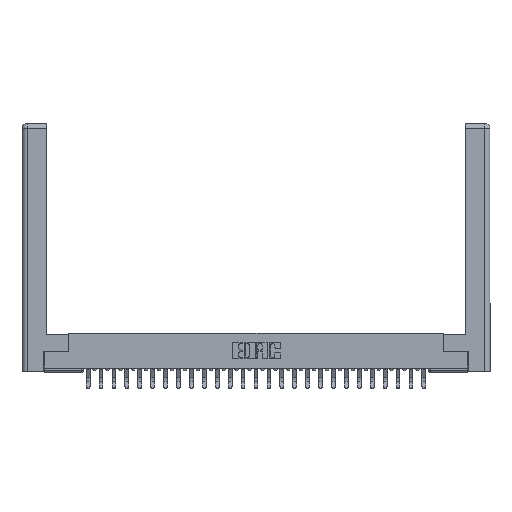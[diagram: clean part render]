
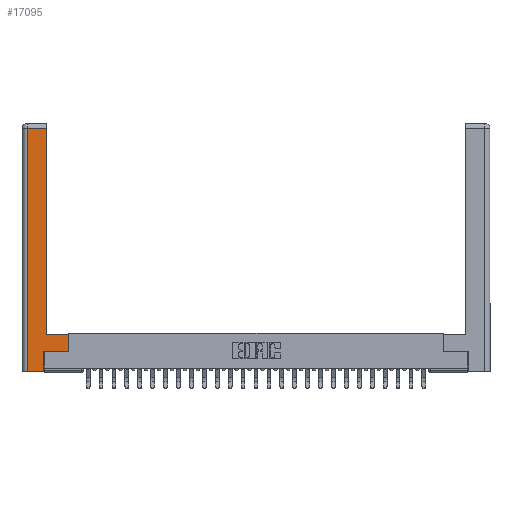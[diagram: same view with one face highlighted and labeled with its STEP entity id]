
A CAD part, top view. The second image highlights one B-rep face of the part: STEP entity #17095.
In plain terms, the highlighted planar face has unit normal (0, 0, 1).
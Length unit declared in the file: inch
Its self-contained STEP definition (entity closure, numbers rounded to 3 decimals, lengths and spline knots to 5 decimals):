
#270 = VECTOR ( 'NONE', #26893, 39.37008 ) ;
#535 = LINE ( 'NONE', #22062, #9933 ) ;
#994 = EDGE_CURVE ( 'NONE', #13343, #8390, #21344, .T. ) ;
#1334 = LINE ( 'NONE', #6790, #270 ) ;
#2785 = CARTESIAN_POINT ( 'NONE',  ( 0.565, 0.245, 0. ) ) ;
#4037 = PLANE ( 'NONE',  #7291 ) ;
#5128 = LINE ( 'NONE', #14419, #5830 ) ;
#5163 = CARTESIAN_POINT ( 'NONE',  ( 0.295, 3., 0. ) ) ;
#5531 = EDGE_CURVE ( 'NONE', #24917, #17816, #5128, .T. ) ;
#5830 = VECTOR ( 'NONE', #5980, 39.37008 ) ;
#5899 = FACE_OUTER_BOUND ( 'NONE', #14785, .T. ) ;
#5980 = DIRECTION ( 'NONE',  ( 0., 1., 0. ) ) ;
#6104 = CARTESIAN_POINT ( 'NONE',  ( 0.295, 0.45, 0. ) ) ;
#6284 = DIRECTION ( 'NONE',  ( 1., 0., 0. ) ) ;
#6790 = CARTESIAN_POINT ( 'NONE',  ( 0.0615, 0., 0. ) ) ;
#6974 = CARTESIAN_POINT ( 'NONE',  ( 0.295, 2.94, 0. ) ) ;
#7065 = CARTESIAN_POINT ( 'NONE',  ( 0.0615, 2.94, 0. ) ) ;
#7217 = DIRECTION ( 'NONE',  ( 0., 1., 0. ) ) ;
#7291 = AXIS2_PLACEMENT_3D ( 'NONE', #19694, #28341, #25826 ) ;
#8374 = ORIENTED_EDGE ( 'NONE', *, *, #19816, .T. ) ;
#8390 = VERTEX_POINT ( 'NONE', #17400 ) ;
#8708 = ORIENTED_EDGE ( 'NONE', *, *, #13750, .T. ) ;
#8835 = LINE ( 'NONE', #19430, #19545 ) ;
#9615 = ORIENTED_EDGE ( 'NONE', *, *, #13649, .T. ) ;
#9900 = ORIENTED_EDGE ( 'NONE', *, *, #17309, .T. ) ;
#9933 = VECTOR ( 'NONE', #26288, 39.37008 ) ;
#10883 = DIRECTION ( 'NONE',  ( -1., 0., 0. ) ) ;
#11458 = ORIENTED_EDGE ( 'NONE', *, *, #994, .T. ) ;
#11755 = CARTESIAN_POINT ( 'NONE',  ( 0.265, 0., 0. ) ) ;
#13343 = VERTEX_POINT ( 'NONE', #14399 ) ;
#13427 = ORIENTED_EDGE ( 'NONE', *, *, #14787, .T. ) ;
#13649 = EDGE_CURVE ( 'NONE', #17816, #25799, #535, .T. ) ;
#13750 = EDGE_CURVE ( 'NONE', #20900, #19204, #23028, .T. ) ;
#14399 = CARTESIAN_POINT ( 'NONE',  ( 0.265, 0., 0. ) ) ;
#14419 = CARTESIAN_POINT ( 'NONE',  ( 0.565, 0.45, 0. ) ) ;
#14785 = EDGE_LOOP ( 'NONE', ( #9900, #8708, #23205, #8374, #11458, #13427, #15799, #9615 ) ) ;
#14787 = EDGE_CURVE ( 'NONE', #8390, #24917, #8835, .T. ) ;
#15225 = CARTESIAN_POINT ( 'NONE',  ( 0.265, 0.245, 0. ) ) ;
#15799 = ORIENTED_EDGE ( 'NONE', *, *, #5531, .T. ) ;
#16006 = CARTESIAN_POINT ( 'NONE',  ( 0.0615, 0., 0. ) ) ;
#17095 = ADVANCED_FACE ( 'NONE', ( #5899 ), #4037, .F. ) ;
#17309 = EDGE_CURVE ( 'NONE', #25799, #20900, #20396, .T. ) ;
#17400 = CARTESIAN_POINT ( 'NONE',  ( 0.265, 0.245, 0. ) ) ;
#17645 = VECTOR ( 'NONE', #7217, 39.37008 ) ;
#17729 = CARTESIAN_POINT ( 'NONE',  ( 0.565, 0.45, 0. ) ) ;
#17816 = VERTEX_POINT ( 'NONE', #17729 ) ;
#18221 = DIRECTION ( 'NONE',  ( 1., 0., 0. ) ) ;
#19204 = VERTEX_POINT ( 'NONE', #7065 ) ;
#19430 = CARTESIAN_POINT ( 'NONE',  ( 0.565, 0.245, 0. ) ) ;
#19544 = LINE ( 'NONE', #11755, #27426 ) ;
#19545 = VECTOR ( 'NONE', #6284, 39.37008 ) ;
#19694 = CARTESIAN_POINT ( 'NONE',  ( 0., 0., 0. ) ) ;
#19816 = EDGE_CURVE ( 'NONE', #26816, #13343, #19544, .T. ) ;
#20396 = LINE ( 'NONE', #5163, #17645 ) ;
#20900 = VERTEX_POINT ( 'NONE', #6974 ) ;
#21019 = VECTOR ( 'NONE', #21672, 39.37008 ) ;
#21344 = LINE ( 'NONE', #15225, #21019 ) ;
#21672 = DIRECTION ( 'NONE',  ( 0., 1., 0. ) ) ;
#22062 = CARTESIAN_POINT ( 'NONE',  ( 0.295, 0.45, 0. ) ) ;
#23028 = LINE ( 'NONE', #26193, #28536 ) ;
#23205 = ORIENTED_EDGE ( 'NONE', *, *, #26066, .T. ) ;
#24917 = VERTEX_POINT ( 'NONE', #2785 ) ;
#25799 = VERTEX_POINT ( 'NONE', #6104 ) ;
#25826 = DIRECTION ( 'NONE',  ( -1., 0., 0. ) ) ;
#26066 = EDGE_CURVE ( 'NONE', #19204, #26816, #1334, .T. ) ;
#26193 = CARTESIAN_POINT ( 'NONE',  ( 0.0615, 2.94, 0. ) ) ;
#26288 = DIRECTION ( 'NONE',  ( -1., 0., 0. ) ) ;
#26816 = VERTEX_POINT ( 'NONE', #16006 ) ;
#26893 = DIRECTION ( 'NONE',  ( 0., -1., 0. ) ) ;
#27426 = VECTOR ( 'NONE', #18221, 39.37008 ) ;
#28341 = DIRECTION ( 'NONE',  ( 0., 0., -1. ) ) ;
#28536 = VECTOR ( 'NONE', #10883, 39.37008 ) ;
